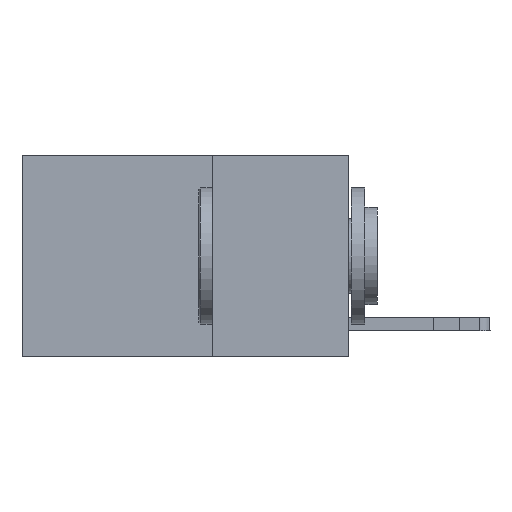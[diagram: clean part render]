
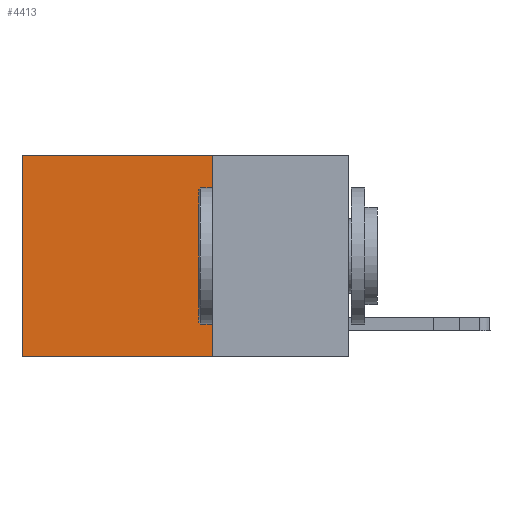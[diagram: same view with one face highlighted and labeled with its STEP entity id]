
A CAD part, left-side view. The second image highlights one B-rep face of the part: STEP entity #4413.
In plain terms, the highlighted planar face has unit normal (-1, 0, 0).
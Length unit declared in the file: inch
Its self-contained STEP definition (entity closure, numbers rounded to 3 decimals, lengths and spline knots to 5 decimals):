
#1434 = VERTEX_POINT ( 'NONE', #20146 ) ;
#1480 = EDGE_CURVE ( 'NONE', #1434, #8010, #18808, .T. ) ;
#2452 = ORIENTED_EDGE ( 'NONE', *, *, #1480, .F. ) ;
#2567 = LINE ( 'NONE', #9888, #5409 ) ;
#3707 = ORIENTED_EDGE ( 'NONE', *, *, #11456, .F. ) ;
#3713 = CARTESIAN_POINT ( 'NONE',  ( 0.2625, 0.6, -0.37 ) ) ;
#4413 = ADVANCED_FACE ( 'NONE', ( #19980 ), #5617, .F. ) ;
#4968 = EDGE_CURVE ( 'NONE', #1434, #7213, #2567, .T. ) ;
#5409 = VECTOR ( 'NONE', #17155, 39.37008 ) ;
#5617 = PLANE ( 'NONE',  #19180 ) ;
#7213 = VERTEX_POINT ( 'NONE', #21663 ) ;
#7525 = DIRECTION ( 'NONE',  ( 1., 0., 0. ) ) ;
#8010 = VERTEX_POINT ( 'NONE', #8644 ) ;
#8644 = CARTESIAN_POINT ( 'NONE',  ( 0.2625, 0.25, -0.37 ) ) ;
#9086 = CARTESIAN_POINT ( 'NONE',  ( 0.2625, 0.25, 0. ) ) ;
#9458 = DIRECTION ( 'NONE',  ( 0., 0., -1. ) ) ;
#9888 = CARTESIAN_POINT ( 'NONE',  ( 0.2625, 0.25, 0. ) ) ;
#10949 = VECTOR ( 'NONE', #17949, 39.37008 ) ;
#11456 = EDGE_CURVE ( 'NONE', #8010, #14107, #21686, .T. ) ;
#11915 = DIRECTION ( 'NONE',  ( 0., 0., -1. ) ) ;
#12161 = CARTESIAN_POINT ( 'NONE',  ( 0.2625, 0.6, 0. ) ) ;
#13056 = CARTESIAN_POINT ( 'NONE',  ( 0.2625, 0.25, 0. ) ) ;
#13464 = VECTOR ( 'NONE', #11915, 39.37008 ) ;
#14107 = VERTEX_POINT ( 'NONE', #3713 ) ;
#14413 = ORIENTED_EDGE ( 'NONE', *, *, #4968, .T. ) ;
#16000 = CARTESIAN_POINT ( 'NONE',  ( 0.2625, 0.25, -0.37 ) ) ;
#16632 = EDGE_CURVE ( 'NONE', #7213, #14107, #18989, .T. ) ;
#17155 = DIRECTION ( 'NONE',  ( 0., 1., 0. ) ) ;
#17949 = DIRECTION ( 'NONE',  ( 0., 1., 0. ) ) ;
#18460 = DIRECTION ( 'NONE',  ( 0., 0., -1. ) ) ;
#18477 = VECTOR ( 'NONE', #18460, 39.37008 ) ;
#18753 = ORIENTED_EDGE ( 'NONE', *, *, #16632, .T. ) ;
#18808 = LINE ( 'NONE', #13056, #18477 ) ;
#18989 = LINE ( 'NONE', #12161, #13464 ) ;
#19180 = AXIS2_PLACEMENT_3D ( 'NONE', #9086, #7525, #9458 ) ;
#19518 = EDGE_LOOP ( 'NONE', ( #18753, #3707, #2452, #14413 ) ) ;
#19980 = FACE_OUTER_BOUND ( 'NONE', #19518, .T. ) ;
#20146 = CARTESIAN_POINT ( 'NONE',  ( 0.2625, 0.25, 0. ) ) ;
#21663 = CARTESIAN_POINT ( 'NONE',  ( 0.2625, 0.6, 0. ) ) ;
#21686 = LINE ( 'NONE', #16000, #10949 ) ;
